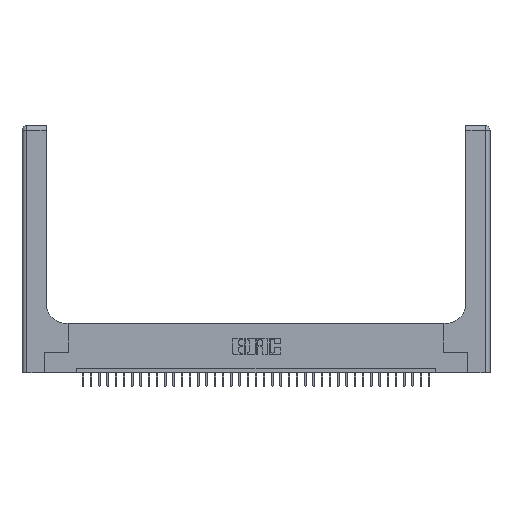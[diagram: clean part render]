
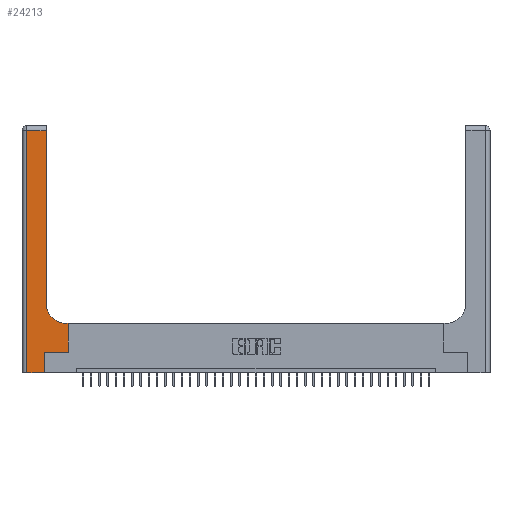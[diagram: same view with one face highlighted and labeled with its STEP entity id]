
A CAD part, top view. The second image highlights one B-rep face of the part: STEP entity #24213.
In plain terms, the highlighted planar face has unit normal (0, 0, 1).
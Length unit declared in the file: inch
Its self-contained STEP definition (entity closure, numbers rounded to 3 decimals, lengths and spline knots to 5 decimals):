
#106 = DIRECTION ( 'NONE',  ( 0., 1., 0. ) ) ;
#113 = LINE ( 'NONE', #35977, #34094 ) ;
#304 = CARTESIAN_POINT ( 'NONE',  ( 0.2915, 0.85, 0.37 ) ) ;
#556 = DIRECTION ( 'NONE',  ( 1., 0., 0. ) ) ;
#1045 = CARTESIAN_POINT ( 'NONE',  ( 0.2915, 3., 0.37 ) ) ;
#1387 = ORIENTED_EDGE ( 'NONE', *, *, #12212, .T. ) ;
#2093 = CARTESIAN_POINT ( 'NONE',  ( 0.2915, 0.6, 0.37 ) ) ;
#2161 = VERTEX_POINT ( 'NONE', #27303 ) ;
#2444 = EDGE_CURVE ( 'NONE', #28998, #27422, #24462, .T. ) ;
#2832 = PLANE ( 'NONE',  #7340 ) ;
#3074 = VERTEX_POINT ( 'NONE', #28838 ) ;
#3168 = DIRECTION ( 'NONE',  ( -1., 0., 0. ) ) ;
#3297 = EDGE_CURVE ( 'NONE', #18237, #29200, #5809, .T. ) ;
#3844 = VECTOR ( 'NONE', #556, 39.37008 ) ;
#3873 = CIRCLE ( 'NONE', #26345, 0.25 ) ;
#5626 = CARTESIAN_POINT ( 'NONE',  ( 0.2915, 2.94, 0.37 ) ) ;
#5661 = LINE ( 'NONE', #35245, #3844 ) ;
#5809 = LINE ( 'NONE', #31737, #25774 ) ;
#6344 = EDGE_CURVE ( 'NONE', #29200, #15250, #16461, .T. ) ;
#6651 = CARTESIAN_POINT ( 'NONE',  ( 0.06, 3., 0.37 ) ) ;
#6940 = VECTOR ( 'NONE', #14211, 39.37008 ) ;
#7340 = AXIS2_PLACEMENT_3D ( 'NONE', #23114, #23342, #17330 ) ;
#8078 = CARTESIAN_POINT ( 'NONE',  ( 0.5415, 0.6, 0.37 ) ) ;
#8344 = CARTESIAN_POINT ( 'NONE',  ( 0.269, 0., 0.37 ) ) ;
#9087 = CARTESIAN_POINT ( 'NONE',  ( 0., 0., 0.37 ) ) ;
#9801 = VECTOR ( 'NONE', #29913, 39.37008 ) ;
#9912 = CARTESIAN_POINT ( 'NONE',  ( 0.5415, 0.85, 0.37 ) ) ;
#10431 = ORIENTED_EDGE ( 'NONE', *, *, #31117, .T. ) ;
#12212 = EDGE_CURVE ( 'NONE', #36313, #18237, #5661, .T. ) ;
#13083 = DIRECTION ( 'NONE',  ( 0., 0., -1. ) ) ;
#13967 = EDGE_CURVE ( 'NONE', #2161, #3074, #36581, .T. ) ;
#14211 = DIRECTION ( 'NONE',  ( 0., 1., 0. ) ) ;
#14390 = DIRECTION ( 'NONE',  ( 1., 0., 0. ) ) ;
#15250 = VERTEX_POINT ( 'NONE', #8078 ) ;
#15392 = FACE_OUTER_BOUND ( 'NONE', #27508, .T. ) ;
#15990 = DIRECTION ( 'NONE',  ( 1., 0., 0. ) ) ;
#16461 = LINE ( 'NONE', #2093, #16949 ) ;
#16949 = VECTOR ( 'NONE', #3168, 39.37008 ) ;
#17330 = DIRECTION ( 'NONE',  ( -1., 0., 0. ) ) ;
#17348 = EDGE_CURVE ( 'NONE', #27422, #2161, #113, .T. ) ;
#17615 = CARTESIAN_POINT ( 'NONE',  ( 0.5585, 0.6, 0.37 ) ) ;
#17926 = ORIENTED_EDGE ( 'NONE', *, *, #3297, .T. ) ;
#18237 = VERTEX_POINT ( 'NONE', #36808 ) ;
#18553 = VECTOR ( 'NONE', #29994, 39.37008 ) ;
#18980 = DIRECTION ( 'NONE',  ( -1., 0., 0. ) ) ;
#20648 = VERTEX_POINT ( 'NONE', #32968 ) ;
#21041 = VECTOR ( 'NONE', #14390, 39.37008 ) ;
#21951 = ORIENTED_EDGE ( 'NONE', *, *, #17348, .T. ) ;
#23114 = CARTESIAN_POINT ( 'NONE',  ( 0., 3., 0.37 ) ) ;
#23342 = DIRECTION ( 'NONE',  ( 0., 0., -1. ) ) ;
#24213 = ADVANCED_FACE ( 'NONE', ( #15392 ), #2832, .F. ) ;
#24462 = LINE ( 'NONE', #1045, #18553 ) ;
#25774 = VECTOR ( 'NONE', #106, 39.37008 ) ;
#26345 = AXIS2_PLACEMENT_3D ( 'NONE', #9912, #13083, #15990 ) ;
#26568 = EDGE_CURVE ( 'NONE', #20648, #36313, #30475, .T. ) ;
#27130 = ORIENTED_EDGE ( 'NONE', *, *, #31303, .T. ) ;
#27303 = CARTESIAN_POINT ( 'NONE',  ( 0.06, 2.94, 0.37 ) ) ;
#27422 = VERTEX_POINT ( 'NONE', #5626 ) ;
#27508 = EDGE_LOOP ( 'NONE', ( #27975, #21951, #33399, #10431, #30956, #1387, #17926, #37259, #27130 ) ) ;
#27975 = ORIENTED_EDGE ( 'NONE', *, *, #2444, .T. ) ;
#28838 = CARTESIAN_POINT ( 'NONE',  ( 0.06, 0., 0.37 ) ) ;
#28998 = VERTEX_POINT ( 'NONE', #304 ) ;
#29200 = VERTEX_POINT ( 'NONE', #17615 ) ;
#29913 = DIRECTION ( 'NONE',  ( 0., -1., 0. ) ) ;
#29994 = DIRECTION ( 'NONE',  ( 0., 1., 0. ) ) ;
#30475 = LINE ( 'NONE', #8344, #6940 ) ;
#30956 = ORIENTED_EDGE ( 'NONE', *, *, #26568, .T. ) ;
#31117 = EDGE_CURVE ( 'NONE', #3074, #20648, #34689, .T. ) ;
#31303 = EDGE_CURVE ( 'NONE', #15250, #28998, #3873, .T. ) ;
#31737 = CARTESIAN_POINT ( 'NONE',  ( 0.5585, 0.25, 0.37 ) ) ;
#32968 = CARTESIAN_POINT ( 'NONE',  ( 0.269, 0., 0.37 ) ) ;
#33399 = ORIENTED_EDGE ( 'NONE', *, *, #13967, .T. ) ;
#33516 = CARTESIAN_POINT ( 'NONE',  ( 0.269, 0.25, 0.37 ) ) ;
#34094 = VECTOR ( 'NONE', #18980, 39.37008 ) ;
#34689 = LINE ( 'NONE', #9087, #21041 ) ;
#35245 = CARTESIAN_POINT ( 'NONE',  ( 0.269, 0.25, 0.37 ) ) ;
#35977 = CARTESIAN_POINT ( 'NONE',  ( 0., 2.94, 0.37 ) ) ;
#36313 = VERTEX_POINT ( 'NONE', #33516 ) ;
#36581 = LINE ( 'NONE', #6651, #9801 ) ;
#36808 = CARTESIAN_POINT ( 'NONE',  ( 0.5585, 0.25, 0.37 ) ) ;
#37259 = ORIENTED_EDGE ( 'NONE', *, *, #6344, .T. ) ;
